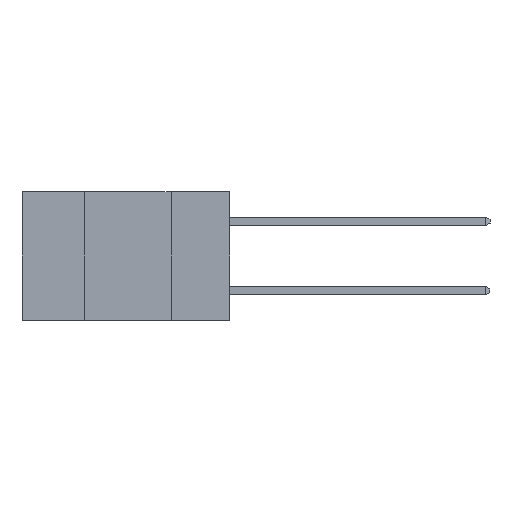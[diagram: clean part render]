
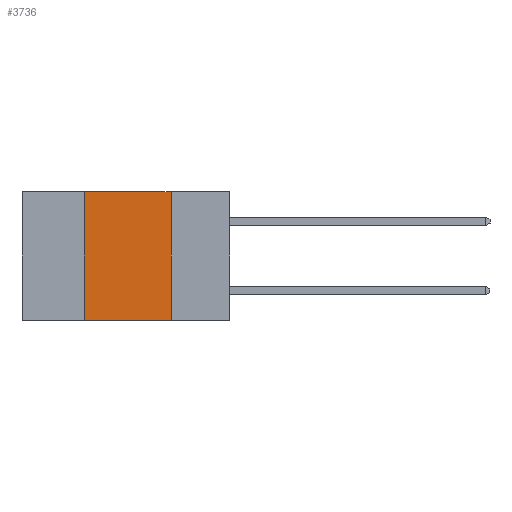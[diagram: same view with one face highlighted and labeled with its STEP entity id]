
A CAD part, left-side view. The second image highlights one B-rep face of the part: STEP entity #3736.
In plain terms, the highlighted planar face has unit normal (-1, 0, 0).
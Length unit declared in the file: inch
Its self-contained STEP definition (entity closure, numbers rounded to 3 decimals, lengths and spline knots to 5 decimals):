
#335 = EDGE_CURVE ( 'NONE', #6644, #7478, #10467, .T. ) ;
#675 = CARTESIAN_POINT ( 'NONE',  ( 0., 0.6, 0. ) ) ;
#710 = ORIENTED_EDGE ( 'NONE', *, *, #335, .F. ) ;
#813 = FACE_OUTER_BOUND ( 'NONE', #12208, .T. ) ;
#897 = VECTOR ( 'NONE', #8527, 39.37008 ) ;
#1432 = AXIS2_PLACEMENT_3D ( 'NONE', #6939, #4945, #2489 ) ;
#2100 = CARTESIAN_POINT ( 'NONE',  ( 0., 0.42, 0. ) ) ;
#2489 = DIRECTION ( 'NONE',  ( 0., 0., -1. ) ) ;
#2897 = CARTESIAN_POINT ( 'NONE',  ( 0., 0.17, 0. ) ) ;
#2947 = DIRECTION ( 'NONE',  ( 0., 0., -1. ) ) ;
#3220 = DIRECTION ( 'NONE',  ( 0., 0., 1. ) ) ;
#3736 = ADVANCED_FACE ( 'NONE', ( #813 ), #6962, .F. ) ;
#4106 = LINE ( 'NONE', #2100, #12773 ) ;
#4945 = DIRECTION ( 'NONE',  ( 1., 0., 0. ) ) ;
#5459 = DIRECTION ( 'NONE',  ( 0., -1., 0. ) ) ;
#5928 = VERTEX_POINT ( 'NONE', #14099 ) ;
#6644 = VERTEX_POINT ( 'NONE', #12007 ) ;
#6670 = CARTESIAN_POINT ( 'NONE',  ( 0., 0.42, 0. ) ) ;
#6939 = CARTESIAN_POINT ( 'NONE',  ( 0., 0.6, 0. ) ) ;
#6962 = PLANE ( 'NONE',  #1432 ) ;
#7478 = VERTEX_POINT ( 'NONE', #12636 ) ;
#8322 = ORIENTED_EDGE ( 'NONE', *, *, #9446, .F. ) ;
#8527 = DIRECTION ( 'NONE',  ( 0., -1., 0. ) ) ;
#9193 = ORIENTED_EDGE ( 'NONE', *, *, #11846, .F. ) ;
#9216 = LINE ( 'NONE', #675, #897 ) ;
#9392 = ORIENTED_EDGE ( 'NONE', *, *, #13900, .T. ) ;
#9446 = EDGE_CURVE ( 'NONE', #5928, #10792, #4106, .T. ) ;
#10153 = VECTOR ( 'NONE', #5459, 39.37008 ) ;
#10467 = LINE ( 'NONE', #2897, #14095 ) ;
#10792 = VERTEX_POINT ( 'NONE', #6670 ) ;
#11846 = EDGE_CURVE ( 'NONE', #10792, #6644, #9216, .T. ) ;
#12007 = CARTESIAN_POINT ( 'NONE',  ( 0., 0.17, 0. ) ) ;
#12208 = EDGE_LOOP ( 'NONE', ( #710, #9193, #8322, #9392 ) ) ;
#12636 = CARTESIAN_POINT ( 'NONE',  ( 0., 0.17, -0.37 ) ) ;
#12773 = VECTOR ( 'NONE', #3220, 39.37008 ) ;
#13099 = LINE ( 'NONE', #14448, #10153 ) ;
#13900 = EDGE_CURVE ( 'NONE', #5928, #7478, #13099, .T. ) ;
#14095 = VECTOR ( 'NONE', #2947, 39.37008 ) ;
#14099 = CARTESIAN_POINT ( 'NONE',  ( 0., 0.42, -0.37 ) ) ;
#14448 = CARTESIAN_POINT ( 'NONE',  ( 0., 0.6, -0.37 ) ) ;
